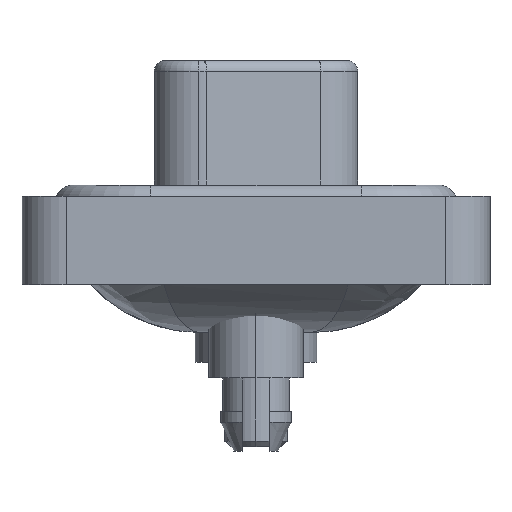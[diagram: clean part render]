
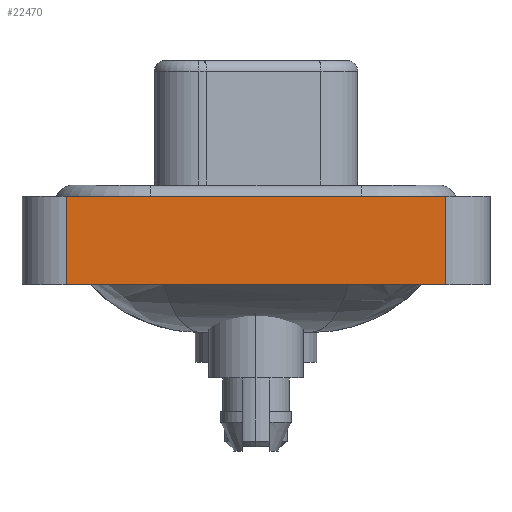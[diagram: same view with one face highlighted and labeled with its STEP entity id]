
A CAD part, left-side view. The second image highlights one B-rep face of the part: STEP entity #22470.
In plain terms, the highlighted planar face has unit normal (-1, 0, 0).
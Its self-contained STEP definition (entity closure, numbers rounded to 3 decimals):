
#658 = VECTOR ( 'NONE', #2510, 1000. ) ;
#934 = CARTESIAN_POINT ( 'NONE',  ( -7.35, 8.55, -3.6 ) ) ;
#1254 = ORIENTED_EDGE ( 'NONE', *, *, #16431, .T. ) ;
#1725 = AXIS2_PLACEMENT_3D ( 'NONE', #19393, #15577, #3257 ) ;
#2185 = VERTEX_POINT ( 'NONE', #12195 ) ;
#2510 = DIRECTION ( 'NONE',  ( 0., -1., 0. ) ) ;
#3257 = DIRECTION ( 'NONE',  ( 0., 0., 1. ) ) ;
#4770 = ORIENTED_EDGE ( 'NONE', *, *, #6588, .F. ) ;
#5970 = VERTEX_POINT ( 'NONE', #11860 ) ;
#6588 = EDGE_CURVE ( 'NONE', #5970, #9711, #18437, .T. ) ;
#6716 = LINE ( 'NONE', #19144, #17206 ) ;
#7163 = CARTESIAN_POINT ( 'NONE',  ( -7.35, -8.55, -3.6 ) ) ;
#7248 = DIRECTION ( 'NONE',  ( 0., -1., 0. ) ) ;
#8338 = DIRECTION ( 'NONE',  ( 0., 0., 1. ) ) ;
#8377 = PLANE ( 'NONE',  #1725 ) ;
#8717 = EDGE_LOOP ( 'NONE', ( #1254, #4770, #16211, #20340 ) ) ;
#8999 = LINE ( 'NONE', #14560, #11965 ) ;
#9711 = VERTEX_POINT ( 'NONE', #21844 ) ;
#11515 = LINE ( 'NONE', #934, #14511 ) ;
#11860 = CARTESIAN_POINT ( 'NONE',  ( -7.35, 8.55, 0.4 ) ) ;
#11965 = VECTOR ( 'NONE', #7248, 1000. ) ;
#12195 = CARTESIAN_POINT ( 'NONE',  ( -7.35, 8.55, -3.6 ) ) ;
#13442 = EDGE_CURVE ( 'NONE', #2185, #5970, #11515, .T. ) ;
#14010 = EDGE_CURVE ( 'NONE', #2185, #21651, #8999, .T. ) ;
#14511 = VECTOR ( 'NONE', #8338, 1000. ) ;
#14560 = CARTESIAN_POINT ( 'NONE',  ( -7.35, -8.55, -3.6 ) ) ;
#15577 = DIRECTION ( 'NONE',  ( -1., 0., 0. ) ) ;
#16211 = ORIENTED_EDGE ( 'NONE', *, *, #13442, .F. ) ;
#16431 = EDGE_CURVE ( 'NONE', #21651, #9711, #6716, .T. ) ;
#17206 = VECTOR ( 'NONE', #19488, 1000. ) ;
#18437 = LINE ( 'NONE', #21901, #658 ) ;
#19144 = CARTESIAN_POINT ( 'NONE',  ( -7.35, -8.55, -3.6 ) ) ;
#19393 = CARTESIAN_POINT ( 'NONE',  ( -7.35, -8.55, -3.6 ) ) ;
#19488 = DIRECTION ( 'NONE',  ( 0., 0., 1. ) ) ;
#20340 = ORIENTED_EDGE ( 'NONE', *, *, #14010, .T. ) ;
#20790 = FACE_OUTER_BOUND ( 'NONE', #8717, .T. ) ;
#21651 = VERTEX_POINT ( 'NONE', #7163 ) ;
#21844 = CARTESIAN_POINT ( 'NONE',  ( -7.35, -8.55, 0.4 ) ) ;
#21901 = CARTESIAN_POINT ( 'NONE',  ( -7.35, -8.55, 0.4 ) ) ;
#22470 = ADVANCED_FACE ( 'NONE', ( #20790 ), #8377, .T. ) ;
